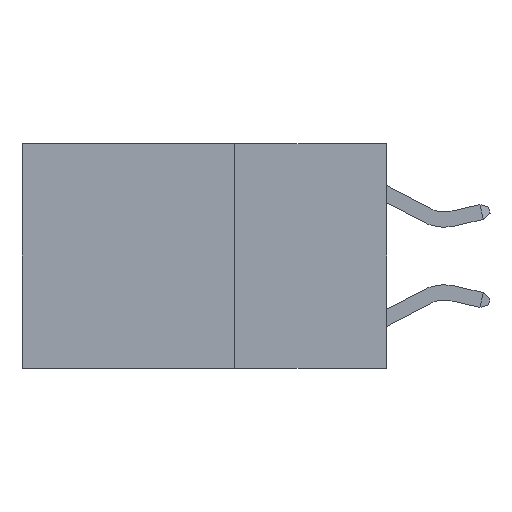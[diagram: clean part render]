
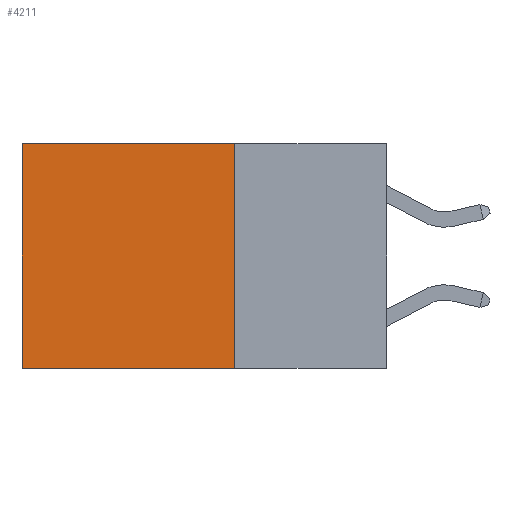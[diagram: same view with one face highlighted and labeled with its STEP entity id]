
A CAD part, left-side view. The second image highlights one B-rep face of the part: STEP entity #4211.
In plain terms, the highlighted planar face has unit normal (-1, 0, 0).
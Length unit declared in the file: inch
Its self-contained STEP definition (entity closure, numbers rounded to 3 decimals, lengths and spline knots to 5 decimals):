
#1019 = ORIENTED_EDGE ( 'NONE', *, *, #19538, .F. ) ;
#1349 = VERTEX_POINT ( 'NONE', #7521 ) ;
#1519 = ORIENTED_EDGE ( 'NONE', *, *, #6919, .F. ) ;
#2172 = LINE ( 'NONE', #9240, #14087 ) ;
#2330 = LINE ( 'NONE', #11761, #17774 ) ;
#2812 = EDGE_CURVE ( 'NONE', #14444, #1349, #2172, .T. ) ;
#3993 = DIRECTION ( 'NONE',  ( 0., 0., -1. ) ) ;
#4147 = VECTOR ( 'NONE', #7349, 39.37008 ) ;
#4211 = ADVANCED_FACE ( 'NONE', ( #7230 ), #8874, .F. ) ;
#5062 = CARTESIAN_POINT ( 'NONE',  ( 0.2625, 0.6, 0. ) ) ;
#5565 = EDGE_LOOP ( 'NONE', ( #16990, #1019, #1519, #9811 ) ) ;
#6902 = VERTEX_POINT ( 'NONE', #17771 ) ;
#6919 = EDGE_CURVE ( 'NONE', #6902, #17963, #2330, .T. ) ;
#7230 = FACE_OUTER_BOUND ( 'NONE', #5565, .T. ) ;
#7349 = DIRECTION ( 'NONE',  ( 0., 1., 0. ) ) ;
#7521 = CARTESIAN_POINT ( 'NONE',  ( 0.2625, 0.6, -0.37 ) ) ;
#7784 = LINE ( 'NONE', #16582, #4147 ) ;
#8874 = PLANE ( 'NONE',  #18793 ) ;
#9240 = CARTESIAN_POINT ( 'NONE',  ( 0.2625, 0.6, 0. ) ) ;
#9548 = CARTESIAN_POINT ( 'NONE',  ( 0.2625, 0.25, 0. ) ) ;
#9811 = ORIENTED_EDGE ( 'NONE', *, *, #17991, .T. ) ;
#10433 = DIRECTION ( 'NONE',  ( 0., 0., -1. ) ) ;
#11109 = DIRECTION ( 'NONE',  ( 0., 1., 0. ) ) ;
#11469 = LINE ( 'NONE', #9548, #19004 ) ;
#11761 = CARTESIAN_POINT ( 'NONE',  ( 0.2625, 0.25, 0. ) ) ;
#12446 = DIRECTION ( 'NONE',  ( 0., 0., -1. ) ) ;
#14078 = CARTESIAN_POINT ( 'NONE',  ( 0.2625, 0.25, -0.37 ) ) ;
#14087 = VECTOR ( 'NONE', #12446, 39.37008 ) ;
#14444 = VERTEX_POINT ( 'NONE', #5062 ) ;
#16536 = CARTESIAN_POINT ( 'NONE',  ( 0.2625, 0.25, 0. ) ) ;
#16582 = CARTESIAN_POINT ( 'NONE',  ( 0.2625, 0.25, -0.37 ) ) ;
#16990 = ORIENTED_EDGE ( 'NONE', *, *, #2812, .T. ) ;
#17771 = CARTESIAN_POINT ( 'NONE',  ( 0.2625, 0.25, 0. ) ) ;
#17774 = VECTOR ( 'NONE', #3993, 39.37008 ) ;
#17963 = VERTEX_POINT ( 'NONE', #14078 ) ;
#17991 = EDGE_CURVE ( 'NONE', #6902, #14444, #11469, .T. ) ;
#18793 = AXIS2_PLACEMENT_3D ( 'NONE', #16536, #19493, #10433 ) ;
#19004 = VECTOR ( 'NONE', #11109, 39.37008 ) ;
#19493 = DIRECTION ( 'NONE',  ( 1., 0., 0. ) ) ;
#19538 = EDGE_CURVE ( 'NONE', #17963, #1349, #7784, .T. ) ;
